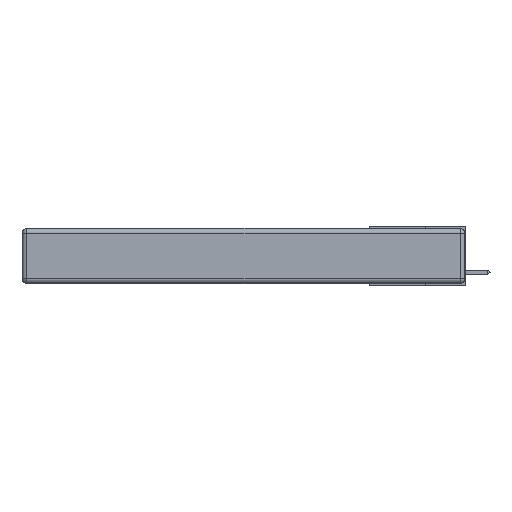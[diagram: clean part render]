
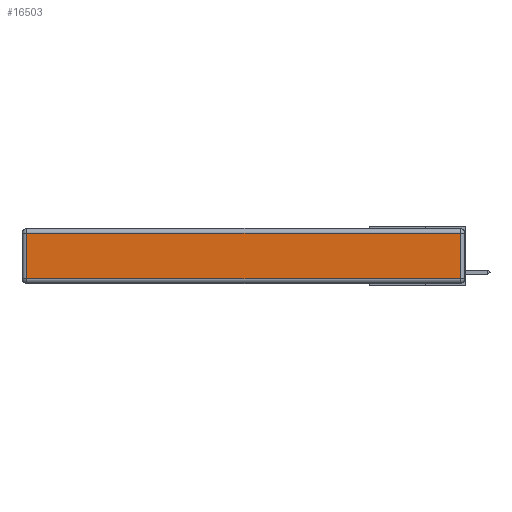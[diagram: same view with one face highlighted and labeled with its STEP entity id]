
A CAD part, left-side view. The second image highlights one B-rep face of the part: STEP entity #16503.
In plain terms, the highlighted planar face has unit normal (-1, 0, 0).
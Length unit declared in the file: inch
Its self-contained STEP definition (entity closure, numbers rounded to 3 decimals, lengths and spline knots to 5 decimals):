
#170 = EDGE_CURVE ( 'NONE', #2898, #1551, #12574, .T. ) ;
#579 = DIRECTION ( 'NONE',  ( 0., 0., 1. ) ) ;
#826 = ORIENTED_EDGE ( 'NONE', *, *, #15918, .T. ) ;
#1491 = VECTOR ( 'NONE', #12266, 39.37008 ) ;
#1547 = ORIENTED_EDGE ( 'NONE', *, *, #16032, .T. ) ;
#1551 = VERTEX_POINT ( 'NONE', #5170 ) ;
#2898 = VERTEX_POINT ( 'NONE', #7166 ) ;
#3084 = ORIENTED_EDGE ( 'NONE', *, *, #9066, .T. ) ;
#3122 = AXIS2_PLACEMENT_3D ( 'NONE', #8832, #7324, #13044 ) ;
#3327 = DIRECTION ( 'NONE',  ( 0., 0., -1. ) ) ;
#5170 = CARTESIAN_POINT ( 'NONE',  ( 0., 2.72, -0.313 ) ) ;
#6384 = VECTOR ( 'NONE', #579, 39.37008 ) ;
#6795 = DIRECTION ( 'NONE',  ( 0., 1., 0. ) ) ;
#7166 = CARTESIAN_POINT ( 'NONE',  ( 0., 2.72, -0.03 ) ) ;
#7324 = DIRECTION ( 'NONE',  ( -1., 0., 0. ) ) ;
#8011 = CARTESIAN_POINT ( 'NONE',  ( 0., 0., -0.313 ) ) ;
#8832 = CARTESIAN_POINT ( 'NONE',  ( 0., 0., -0.343 ) ) ;
#8954 = LINE ( 'NONE', #17387, #14081 ) ;
#9066 = EDGE_CURVE ( 'NONE', #1551, #10997, #17775, .T. ) ;
#9130 = CARTESIAN_POINT ( 'NONE',  ( 0., 0.03, -0.03 ) ) ;
#9438 = CARTESIAN_POINT ( 'NONE',  ( 0., 0.03, -0.343 ) ) ;
#10192 = PLANE ( 'NONE',  #3122 ) ;
#10530 = EDGE_LOOP ( 'NONE', ( #3084, #826, #1547, #13509 ) ) ;
#10752 = FACE_OUTER_BOUND ( 'NONE', #10530, .T. ) ;
#10997 = VERTEX_POINT ( 'NONE', #14456 ) ;
#12266 = DIRECTION ( 'NONE',  ( 0., -1., 0. ) ) ;
#12574 = LINE ( 'NONE', #16587, #18181 ) ;
#12774 = VERTEX_POINT ( 'NONE', #9130 ) ;
#13044 = DIRECTION ( 'NONE',  ( 0., 0., 1. ) ) ;
#13509 = ORIENTED_EDGE ( 'NONE', *, *, #170, .T. ) ;
#14081 = VECTOR ( 'NONE', #6795, 39.37008 ) ;
#14456 = CARTESIAN_POINT ( 'NONE',  ( 0., 0.03, -0.313 ) ) ;
#15918 = EDGE_CURVE ( 'NONE', #10997, #12774, #18502, .T. ) ;
#16032 = EDGE_CURVE ( 'NONE', #12774, #2898, #8954, .T. ) ;
#16503 = ADVANCED_FACE ( 'NONE', ( #10752 ), #10192, .T. ) ;
#16587 = CARTESIAN_POINT ( 'NONE',  ( 0., 2.72, -0.343 ) ) ;
#17387 = CARTESIAN_POINT ( 'NONE',  ( 0., 2.75, -0.03 ) ) ;
#17775 = LINE ( 'NONE', #8011, #1491 ) ;
#18181 = VECTOR ( 'NONE', #3327, 39.37008 ) ;
#18502 = LINE ( 'NONE', #9438, #6384 ) ;
